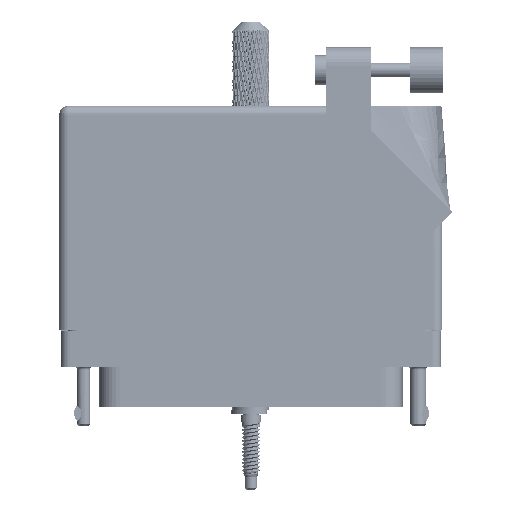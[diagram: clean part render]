
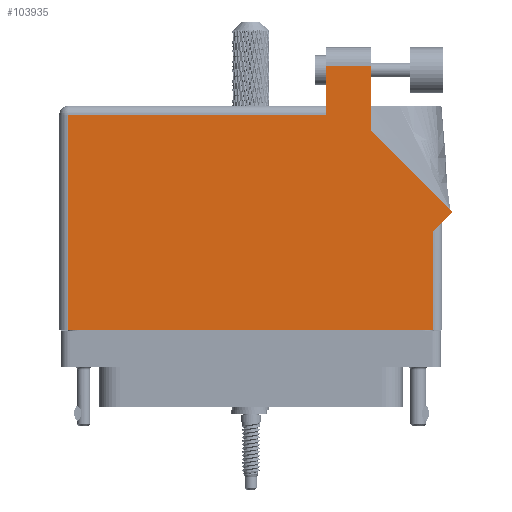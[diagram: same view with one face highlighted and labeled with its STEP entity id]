
A CAD part, front view. The second image highlights one B-rep face of the part: STEP entity #103935.
In plain terms, the highlighted face is planar.
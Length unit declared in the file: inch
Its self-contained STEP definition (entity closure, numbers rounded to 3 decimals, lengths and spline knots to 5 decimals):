
#1423 = DIRECTION ( 'NONE',  ( -1., 0., 0. ) ) ;
#3480 = LINE ( 'NONE', #13729, #35745 ) ;
#13729 = CARTESIAN_POINT ( 'NONE',  ( -1.306, 1.368, 0.455 ) ) ;
#14313 = EDGE_CURVE ( 'NONE', #104147, #122520, #79570, .T. ) ;
#15774 = VERTEX_POINT ( 'NONE', #27406 ) ;
#18368 = CARTESIAN_POINT ( 'NONE',  ( 0.513, 1.43, 0.455 ) ) ;
#19844 = CARTESIAN_POINT ( 'NONE',  ( 1.244, 0.575, 0.455 ) ) ;
#20373 = ORIENTED_EDGE ( 'NONE', *, *, #14313, .T. ) ;
#23540 = DIRECTION ( 'NONE',  ( -1., 0., 0. ) ) ;
#24932 = VECTOR ( 'NONE', #25934, 39.37008 ) ;
#24998 = CARTESIAN_POINT ( 'NONE',  ( -1.306, 1.43, 0.455 ) ) ;
#25934 = DIRECTION ( 'NONE',  ( 0., 1., 0. ) ) ;
#26513 = EDGE_CURVE ( 'NONE', #122520, #35883, #57706, .T. ) ;
#27406 = CARTESIAN_POINT ( 'NONE',  ( 1.37671, 0.70771, 0.455 ) ) ;
#27689 = ORIENTED_EDGE ( 'NONE', *, *, #58569, .T. ) ;
#28090 = VECTOR ( 'NONE', #119580, 39.37008 ) ;
#30210 = LINE ( 'NONE', #88390, #83715 ) ;
#31087 = LINE ( 'NONE', #93131, #24932 ) ;
#33759 = ORIENTED_EDGE ( 'NONE', *, *, #69186, .T. ) ;
#33963 = EDGE_LOOP ( 'NONE', ( #27689, #20373, #46946, #41449, #92927, #33759, #50772, #89902, #52205 ) ) ;
#34676 = VERTEX_POINT ( 'NONE', #107106 ) ;
#35745 = VECTOR ( 'NONE', #23540, 39.37008 ) ;
#35883 = VERTEX_POINT ( 'NONE', #66828 ) ;
#41449 = ORIENTED_EDGE ( 'NONE', *, *, #65622, .T. ) ;
#44258 = DIRECTION ( 'NONE',  ( 0., 0., -1. ) ) ;
#44330 = VECTOR ( 'NONE', #1423, 39.37008 ) ;
#44828 = CARTESIAN_POINT ( 'NONE',  ( 0.513, 1.705, 0.455 ) ) ;
#46946 = ORIENTED_EDGE ( 'NONE', *, *, #26513, .T. ) ;
#47604 = LINE ( 'NONE', #73771, #64388 ) ;
#49638 = DIRECTION ( 'NONE',  ( 0., -1., 0. ) ) ;
#50772 = ORIENTED_EDGE ( 'NONE', *, *, #57465, .T. ) ;
#51156 = DIRECTION ( 'NONE',  ( -0.707, 0.707, 0. ) ) ;
#52205 = ORIENTED_EDGE ( 'NONE', *, *, #53688, .T. ) ;
#52671 = FACE_OUTER_BOUND ( 'NONE', #33963, .T. ) ;
#53688 = EDGE_CURVE ( 'NONE', #15774, #57858, #30210, .T. ) ;
#54513 = DIRECTION ( 'NONE',  ( -1., 0., 0. ) ) ;
#57465 = EDGE_CURVE ( 'NONE', #66685, #60800, #64939, .T. ) ;
#57706 = LINE ( 'NONE', #18368, #120472 ) ;
#57858 = VERTEX_POINT ( 'NONE', #67668 ) ;
#58569 = EDGE_CURVE ( 'NONE', #57858, #104147, #31087, .T. ) ;
#60800 = VERTEX_POINT ( 'NONE', #19844 ) ;
#64388 = VECTOR ( 'NONE', #101633, 39.37008 ) ;
#64939 = LINE ( 'NONE', #90499, #28090 ) ;
#65622 = EDGE_CURVE ( 'NONE', #35883, #118397, #3480, .T. ) ;
#66685 = VERTEX_POINT ( 'NONE', #81030 ) ;
#66828 = CARTESIAN_POINT ( 'NONE',  ( 0.513, 1.368, 0.455 ) ) ;
#67668 = CARTESIAN_POINT ( 'NONE',  ( 0.82, 1.26442, 0.455 ) ) ;
#69186 = EDGE_CURVE ( 'NONE', #34676, #66685, #110210, .T. ) ;
#69252 = AXIS2_PLACEMENT_3D ( 'NONE', #24998, #44258, #54513 ) ;
#73771 = CARTESIAN_POINT ( 'NONE',  ( -1.244, -0.1, 0.455 ) ) ;
#73986 = CARTESIAN_POINT ( 'NONE',  ( -1.306, -0.1, 0.455 ) ) ;
#77191 = VECTOR ( 'NONE', #82813, 39.37008 ) ;
#79570 = LINE ( 'NONE', #89161, #44330 ) ;
#81030 = CARTESIAN_POINT ( 'NONE',  ( 1.244, -0.1, 0.455 ) ) ;
#82813 = DIRECTION ( 'NONE',  ( 0.707, 0.707, 0. ) ) ;
#83715 = VECTOR ( 'NONE', #51156, 39.37008 ) ;
#88390 = CARTESIAN_POINT ( 'NONE',  ( 1.37671, 0.70771, 0.455 ) ) ;
#88715 = VECTOR ( 'NONE', #112518, 39.37008 ) ;
#89161 = CARTESIAN_POINT ( 'NONE',  ( 0.513, 1.705, 0.455 ) ) ;
#89902 = ORIENTED_EDGE ( 'NONE', *, *, #125458, .T. ) ;
#90499 = CARTESIAN_POINT ( 'NONE',  ( 1.244, 0.637, 0.455 ) ) ;
#90715 = CARTESIAN_POINT ( 'NONE',  ( -1.244, 1.368, 0.455 ) ) ;
#92927 = ORIENTED_EDGE ( 'NONE', *, *, #112896, .T. ) ;
#93131 = CARTESIAN_POINT ( 'NONE',  ( 0.82, 1.26442, 0.455 ) ) ;
#101633 = DIRECTION ( 'NONE',  ( 0., -1., 0. ) ) ;
#102134 = CARTESIAN_POINT ( 'NONE',  ( 1.306, 0.637, 0.455 ) ) ;
#102950 = PLANE ( 'NONE',  #69252 ) ;
#103285 = LINE ( 'NONE', #102134, #77191 ) ;
#103935 = ADVANCED_FACE ( 'NONE', ( #52671 ), #102950, .F. ) ;
#104147 = VERTEX_POINT ( 'NONE', #109223 ) ;
#107106 = CARTESIAN_POINT ( 'NONE',  ( -1.244, -0.1, 0.455 ) ) ;
#109223 = CARTESIAN_POINT ( 'NONE',  ( 0.82, 1.705, 0.455 ) ) ;
#110210 = LINE ( 'NONE', #73986, #88715 ) ;
#112518 = DIRECTION ( 'NONE',  ( 1., 0., 0. ) ) ;
#112896 = EDGE_CURVE ( 'NONE', #118397, #34676, #47604, .T. ) ;
#118397 = VERTEX_POINT ( 'NONE', #90715 ) ;
#119580 = DIRECTION ( 'NONE',  ( 0., 1., 0. ) ) ;
#120472 = VECTOR ( 'NONE', #49638, 39.37008 ) ;
#122520 = VERTEX_POINT ( 'NONE', #44828 ) ;
#125458 = EDGE_CURVE ( 'NONE', #60800, #15774, #103285, .T. ) ;
